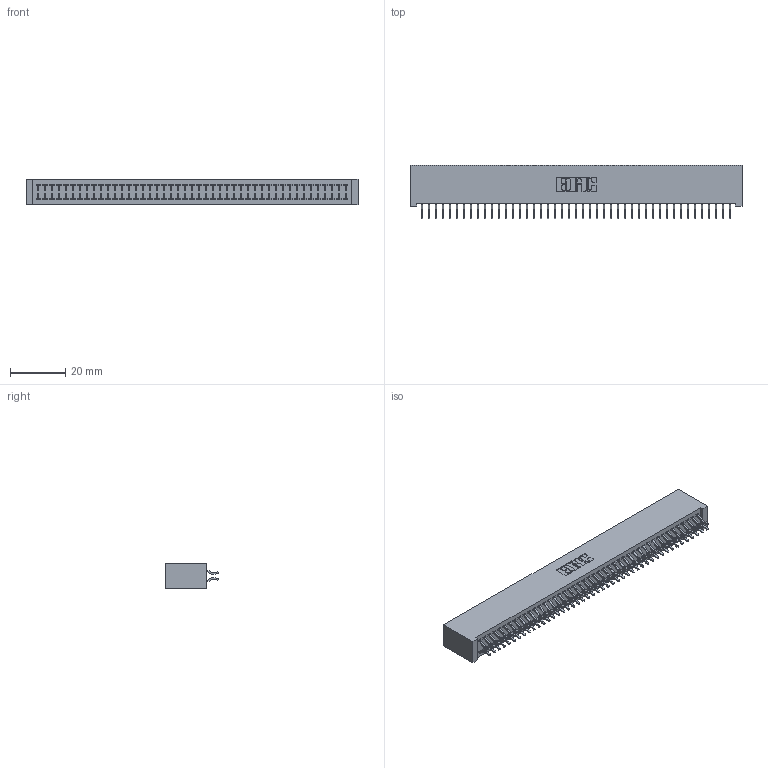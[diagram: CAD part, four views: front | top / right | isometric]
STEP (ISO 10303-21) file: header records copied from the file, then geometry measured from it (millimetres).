
FILE_DESCRIPTION (( 'STEP AP203' ), '1' );
FILE_NAME ('342-090-556-201.STEP', '2018-08-14T01:19:37', ( '' ), ( '' ), 'SwSTEP 2.0', 'SolidWorks 2016', '' );
FILE_SCHEMA (( 'CONFIG_CONTROL_DESIGN' ));
Length unit declared in the file: inch
Products named in the file (3): 342 Part_Lugless; 345-292-001_556 Tail; 342-090-556-201
Assembly tree (91 placements, depth 2):
  342-090-556-201
    342 Part_Lugless
    345-292-001_556 Tail  x90
Bounding box: 120.55 x 19.58 x 9.4 mm (x, y, z)
Volume: 11282.7 mm3; surface area: 18798.2 mm2
Topology: 91 solids, 91 shells, 5322 faces, 15845 edges, 10442 vertices
Faces by surface type: plane 3662, cylinder 1660
Entity records: 28373 total; most frequent: CARTESIAN_POINT 4710, ORIENTED_EDGE 4634, DIRECTION 4001, EDGE_CURVE 2317, LINE 2189, VECTOR 2189, VERTEX_POINT 1542, AXIS2_PLACEMENT_3D 906
